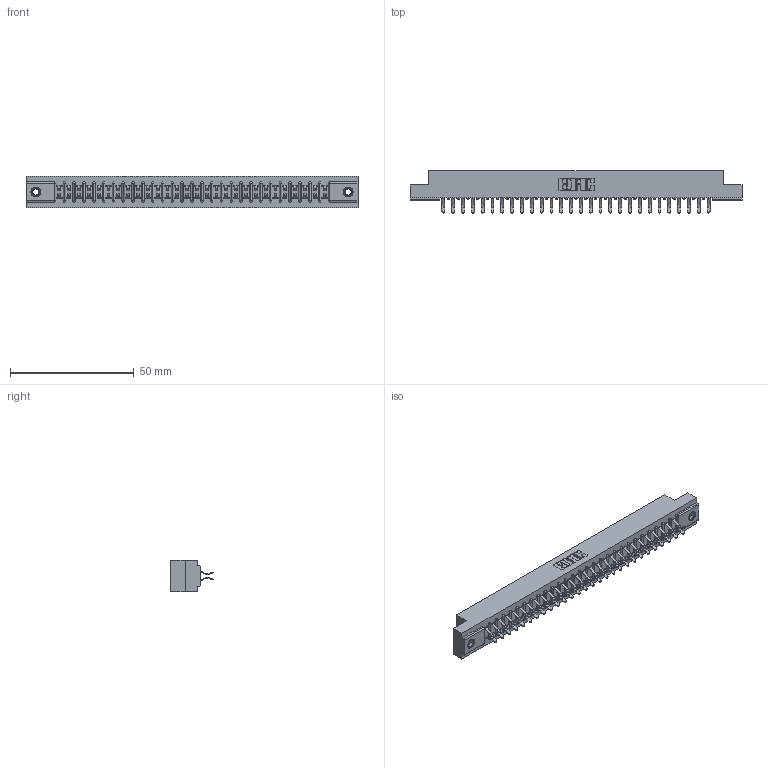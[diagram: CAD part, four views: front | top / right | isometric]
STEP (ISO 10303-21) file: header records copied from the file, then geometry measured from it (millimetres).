
FILE_DESCRIPTION (( 'STEP AP203' ), '1' );
FILE_NAME ('357-056-556-207.STEP', '2018-08-11T18:01:33', ( '' ), ( '' ), 'SwSTEP 2.0', 'SolidWorks 2016', '' );
FILE_SCHEMA (( 'CONFIG_CONTROL_DESIGN' ));
Length unit declared in the file: inch
Products named in the file (4): 307 Part_.156 Dia Mounting Holes; 307-290-001_556; 345-250-001_345-250-005-103; 357-056-556-207
Assembly tree (59 placements, depth 2):
  357-056-556-207
    307 Part_.156 Dia Mounting Holes
    307-290-001_556  x56
    345-250-001_345-250-005-103  x2
Bounding box: 133.96 x 16.97 x 12.7 mm (x, y, z)
Volume: 14122.1 mm3; surface area: 16882.4 mm2
Topology: 59 solids, 59 shells, 3007 faces, 8411 edges, 5446 vertices
Faces by surface type: plane 1950, cylinder 983, sphere 58, cone 12, torus 4
Entity records: 27915 total; most frequent: CARTESIAN_POINT 4555, ORIENTED_EDGE 4506, DIRECTION 4477, EDGE_CURVE 2253, LINE 1721, VECTOR 1721, VERTEX_POINT 1456, AXIS2_PLACEMENT_3D 1378
